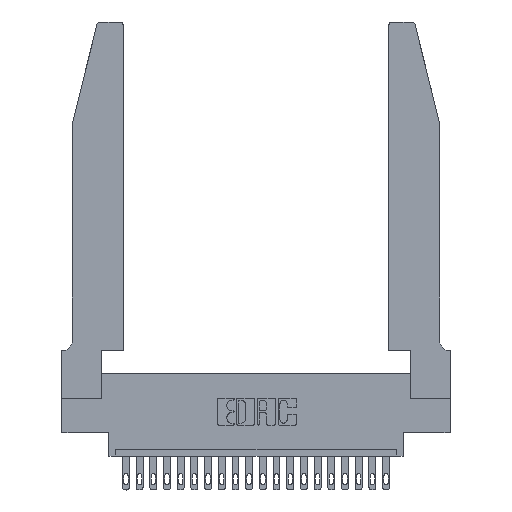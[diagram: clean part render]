
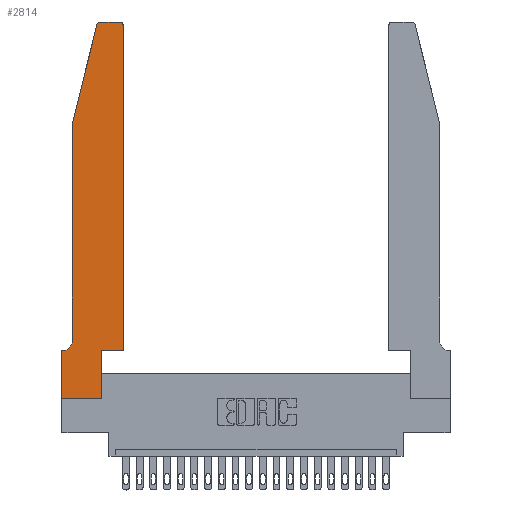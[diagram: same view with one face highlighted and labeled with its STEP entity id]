
A CAD part, top view. The second image highlights one B-rep face of the part: STEP entity #2814.
In plain terms, the highlighted planar face has unit normal (0, 0, 1).
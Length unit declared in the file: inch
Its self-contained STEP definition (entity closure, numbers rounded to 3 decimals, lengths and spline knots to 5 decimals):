
#72 = CARTESIAN_POINT ( 'NONE',  ( 0., 0., 0.37 ) ) ;
#240 = EDGE_CURVE ( 'NONE', #7819, #22164, #4862, .T. ) ;
#359 = LINE ( 'NONE', #17734, #8888 ) ;
#554 = ORIENTED_EDGE ( 'NONE', *, *, #4041, .T. ) ;
#567 = ORIENTED_EDGE ( 'NONE', *, *, #1457, .T. ) ;
#697 = AXIS2_PLACEMENT_3D ( 'NONE', #22461, #5050, #18841 ) ;
#953 = LINE ( 'NONE', #12007, #5658 ) ;
#1170 = CARTESIAN_POINT ( 'NONE',  ( 0.0055, 0.42, 0.37 ) ) ;
#1457 = EDGE_CURVE ( 'NONE', #2718, #20235, #953, .T. ) ;
#1538 = CARTESIAN_POINT ( 'NONE',  ( 0.0055, 0.35, 0.37 ) ) ;
#1588 = LINE ( 'NONE', #6354, #19784 ) ;
#1923 = ORIENTED_EDGE ( 'NONE', *, *, #3791, .T. ) ;
#2209 = EDGE_CURVE ( 'NONE', #22164, #9070, #7801, .T. ) ;
#2624 = EDGE_CURVE ( 'NONE', #4952, #7819, #359, .T. ) ;
#2718 = VERTEX_POINT ( 'NONE', #4109 ) ;
#2814 = ADVANCED_FACE ( 'NONE', ( #6124 ), #4405, .T. ) ;
#3064 = CARTESIAN_POINT ( 'NONE',  ( 0.2865, 0., 0.37 ) ) ;
#3154 = DIRECTION ( 'NONE',  ( -1., 0., 0. ) ) ;
#3419 = CARTESIAN_POINT ( 'NONE',  ( 0., 0., 0.37 ) ) ;
#3563 = CARTESIAN_POINT ( 'NONE',  ( 0.0755, 2., 0.37 ) ) ;
#3791 = EDGE_CURVE ( 'NONE', #9174, #2718, #19022, .T. ) ;
#4041 = EDGE_CURVE ( 'NONE', #13399, #9174, #12672, .T. ) ;
#4088 = ORIENTED_EDGE ( 'NONE', *, *, #2624, .T. ) ;
#4109 = CARTESIAN_POINT ( 'NONE',  ( 0.4205, 2.75, 0.37 ) ) ;
#4405 = PLANE ( 'NONE',  #20582 ) ;
#4408 = EDGE_CURVE ( 'NONE', #9070, #4617, #22858, .T. ) ;
#4617 = VERTEX_POINT ( 'NONE', #13307 ) ;
#4862 = LINE ( 'NONE', #10876, #9806 ) ;
#4896 = CARTESIAN_POINT ( 'NONE',  ( 0.0755, 0.42, 0.37 ) ) ;
#4948 = VECTOR ( 'NONE', #15529, 39.37008 ) ;
#4952 = VERTEX_POINT ( 'NONE', #1538 ) ;
#5017 = DIRECTION ( 'NONE',  ( 0., 0., -1. ) ) ;
#5050 = DIRECTION ( 'NONE',  ( 0., 0., 1. ) ) ;
#5206 = CARTESIAN_POINT ( 'NONE',  ( 0.4505, 2.72, 0.37 ) ) ;
#5264 = CARTESIAN_POINT ( 'NONE',  ( 0.4205, 2.72, 0.37 ) ) ;
#5274 = ORIENTED_EDGE ( 'NONE', *, *, #240, .T. ) ;
#5509 = VERTEX_POINT ( 'NONE', #4896 ) ;
#5658 = VECTOR ( 'NONE', #15597, 39.37008 ) ;
#6124 = FACE_OUTER_BOUND ( 'NONE', #7171, .T. ) ;
#6354 = CARTESIAN_POINT ( 'NONE',  ( 0.0755, 2., 0.37 ) ) ;
#6625 = CIRCLE ( 'NONE', #697, 0.03 ) ;
#6678 = CARTESIAN_POINT ( 'NONE',  ( 0.284, 2.75, 0.37 ) ) ;
#6995 = ORIENTED_EDGE ( 'NONE', *, *, #22631, .T. ) ;
#7171 = EDGE_LOOP ( 'NONE', ( #567, #18301, #19249, #8251, #6995, #4088, #5274, #19238, #11020, #16622, #554, #1923 ) ) ;
#7801 = LINE ( 'NONE', #72, #15452 ) ;
#7819 = VERTEX_POINT ( 'NONE', #12708 ) ;
#7870 = CARTESIAN_POINT ( 'NONE',  ( 0., 0.35, 0.37 ) ) ;
#7881 = DIRECTION ( 'NONE',  ( 0., 1., 0. ) ) ;
#7938 = EDGE_CURVE ( 'NONE', #4617, #13399, #14273, .T. ) ;
#8167 = AXIS2_PLACEMENT_3D ( 'NONE', #1170, #5017, #3154 ) ;
#8251 = ORIENTED_EDGE ( 'NONE', *, *, #18778, .T. ) ;
#8575 = CARTESIAN_POINT ( 'NONE',  ( 0.2865, 0.35, 0.37 ) ) ;
#8888 = VECTOR ( 'NONE', #18202, 39.37008 ) ;
#9070 = VERTEX_POINT ( 'NONE', #3064 ) ;
#9174 = VERTEX_POINT ( 'NONE', #5206 ) ;
#9461 = VECTOR ( 'NONE', #11582, 39.37008 ) ;
#9806 = VECTOR ( 'NONE', #14000, 39.37008 ) ;
#9865 = VECTOR ( 'NONE', #20669, 39.37008 ) ;
#9902 = CARTESIAN_POINT ( 'NONE',  ( 0.4505, 0.35, 0.37 ) ) ;
#10287 = CARTESIAN_POINT ( 'NONE',  ( 0.4505, 0.35, 0.37 ) ) ;
#10876 = CARTESIAN_POINT ( 'NONE',  ( 0., 0., 0.37 ) ) ;
#11020 = ORIENTED_EDGE ( 'NONE', *, *, #4408, .T. ) ;
#11326 = DIRECTION ( 'NONE',  ( 0., 0., 1. ) ) ;
#11582 = DIRECTION ( 'NONE',  ( -0.239, -0.971, 0. ) ) ;
#12007 = CARTESIAN_POINT ( 'NONE',  ( 0.2605, 2.75, 0.37 ) ) ;
#12645 = CARTESIAN_POINT ( 'NONE',  ( 0.4505, 0.35, 0.37 ) ) ;
#12672 = LINE ( 'NONE', #12645, #13213 ) ;
#12708 = CARTESIAN_POINT ( 'NONE',  ( 0., 0.35, 0.37 ) ) ;
#13213 = VECTOR ( 'NONE', #7881, 39.37008 ) ;
#13307 = CARTESIAN_POINT ( 'NONE',  ( 0.2865, 0.35, 0.37 ) ) ;
#13324 = EDGE_CURVE ( 'NONE', #20235, #14539, #6625, .T. ) ;
#13340 = CIRCLE ( 'NONE', #8167, 0.07 ) ;
#13399 = VERTEX_POINT ( 'NONE', #10287 ) ;
#14000 = DIRECTION ( 'NONE',  ( 0., -1., 0. ) ) ;
#14273 = LINE ( 'NONE', #9902, #9865 ) ;
#14539 = VERTEX_POINT ( 'NONE', #15958 ) ;
#15452 = VECTOR ( 'NONE', #15654, 39.37008 ) ;
#15529 = DIRECTION ( 'NONE',  ( 0., 1., 0. ) ) ;
#15597 = DIRECTION ( 'NONE',  ( -1., 0., 0. ) ) ;
#15654 = DIRECTION ( 'NONE',  ( 1., 0., 0. ) ) ;
#15709 = EDGE_CURVE ( 'NONE', #14539, #21042, #21850, .T. ) ;
#15958 = CARTESIAN_POINT ( 'NONE',  ( 0.25487, 2.72718, 0.37 ) ) ;
#16622 = ORIENTED_EDGE ( 'NONE', *, *, #7938, .T. ) ;
#16772 = DIRECTION ( 'NONE',  ( 1., 0., 0. ) ) ;
#17482 = DIRECTION ( 'NONE',  ( 1., 0., 0. ) ) ;
#17734 = CARTESIAN_POINT ( 'NONE',  ( 0.0755, 0.35, 0.37 ) ) ;
#18202 = DIRECTION ( 'NONE',  ( -1., 0., 0. ) ) ;
#18301 = ORIENTED_EDGE ( 'NONE', *, *, #13324, .T. ) ;
#18626 = CARTESIAN_POINT ( 'NONE',  ( 0.0755, 2., 0.37 ) ) ;
#18778 = EDGE_CURVE ( 'NONE', #21042, #5509, #1588, .T. ) ;
#18841 = DIRECTION ( 'NONE',  ( 1., 0., 0. ) ) ;
#19022 = CIRCLE ( 'NONE', #19288, 0.03 ) ;
#19198 = DIRECTION ( 'NONE',  ( 0., 0., 1. ) ) ;
#19238 = ORIENTED_EDGE ( 'NONE', *, *, #2209, .T. ) ;
#19249 = ORIENTED_EDGE ( 'NONE', *, *, #15709, .T. ) ;
#19288 = AXIS2_PLACEMENT_3D ( 'NONE', #5264, #19198, #17482 ) ;
#19784 = VECTOR ( 'NONE', #20658, 39.37008 ) ;
#20235 = VERTEX_POINT ( 'NONE', #6678 ) ;
#20582 = AXIS2_PLACEMENT_3D ( 'NONE', #7870, #11326, #16772 ) ;
#20658 = DIRECTION ( 'NONE',  ( 0., -1., 0. ) ) ;
#20669 = DIRECTION ( 'NONE',  ( 1., 0., 0. ) ) ;
#21042 = VERTEX_POINT ( 'NONE', #3563 ) ;
#21850 = LINE ( 'NONE', #18626, #9461 ) ;
#22164 = VERTEX_POINT ( 'NONE', #3419 ) ;
#22461 = CARTESIAN_POINT ( 'NONE',  ( 0.284, 2.72, 0.37 ) ) ;
#22631 = EDGE_CURVE ( 'NONE', #5509, #4952, #13340, .T. ) ;
#22858 = LINE ( 'NONE', #8575, #4948 ) ;
